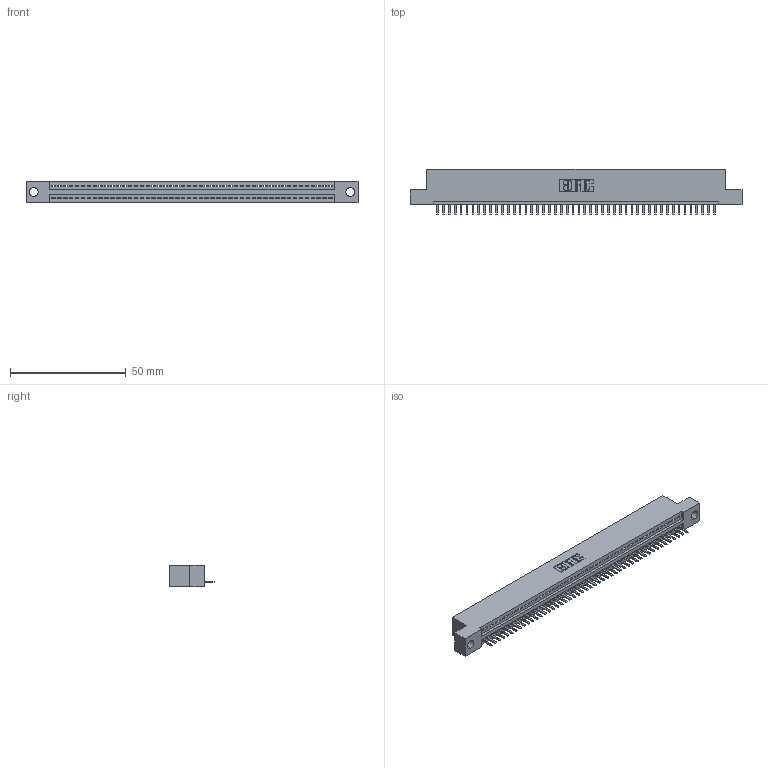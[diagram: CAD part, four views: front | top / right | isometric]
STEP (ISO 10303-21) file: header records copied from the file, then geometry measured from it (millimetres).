
FILE_DESCRIPTION (( 'STEP AP203' ), '1' );
FILE_NAME ('345-048-520-104.STEP', '2019-10-09T04:02:56', ( '' ), ( '' ), 'SwSTEP 2.0', 'SolidWorks 2016', '' );
FILE_SCHEMA (( 'CONFIG_CONTROL_DESIGN' ));
Length unit declared in the file: inch
Products named in the file (3): 345-292-001_345-293-120; 345-048-520-104; 345 Part_Flush Mounting Lugs - 0.156 Dia-TH
Assembly tree (49 placements, depth 2):
  345-048-520-104
    345 Part_Flush Mounting Lugs - 0.156 Dia-TH
    345-292-001_345-293-120  x48
Bounding box: 143.13 x 19.68 x 9.4 mm (x, y, z)
Volume: 13417.8 mm3; surface area: 17269.6 mm2
Topology: 49 solids, 49 shells, 3102 faces, 9173 edges, 5986 vertices
Faces by surface type: plane 2096, cylinder 1006
Entity records: 35435 total; most frequent: CARTESIAN_POINT 6156, ORIENTED_EDGE 6126, DIRECTION 5355, EDGE_CURVE 3063, VECTOR 2735, LINE 2735, VERTEX_POINT 2038, AXIS2_PLACEMENT_3D 1310
